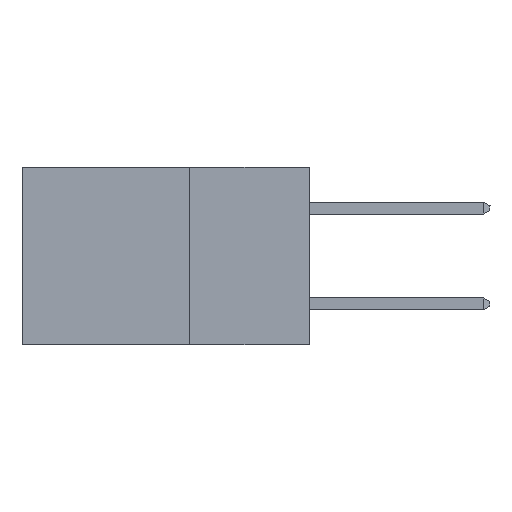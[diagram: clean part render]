
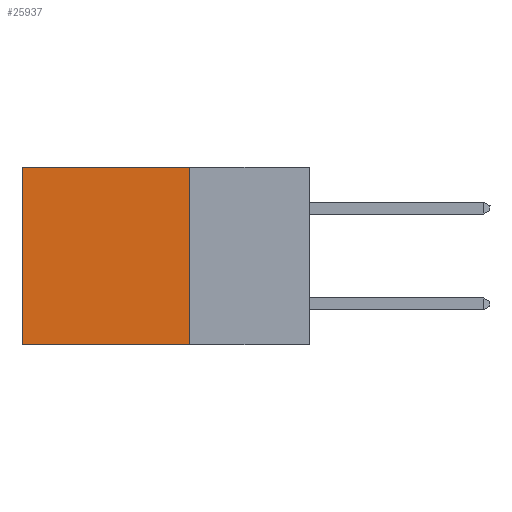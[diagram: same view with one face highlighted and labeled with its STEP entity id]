
A CAD part, left-side view. The second image highlights one B-rep face of the part: STEP entity #25937.
In plain terms, the highlighted planar face has unit normal (-1, 0, 0).
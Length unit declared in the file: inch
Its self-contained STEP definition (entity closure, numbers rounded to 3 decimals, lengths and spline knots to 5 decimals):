
#887 = CARTESIAN_POINT ( 'NONE',  ( 0.2875, 0.25, 0. ) ) ;
#1950 = ORIENTED_EDGE ( 'NONE', *, *, #26668, .T. ) ;
#3660 = VECTOR ( 'NONE', #9837, 39.37008 ) ;
#6089 = EDGE_LOOP ( 'NONE', ( #31651, #23445, #15023, #1950 ) ) ;
#6112 = LINE ( 'NONE', #8741, #6908 ) ;
#6908 = VECTOR ( 'NONE', #26949, 39.37008 ) ;
#7460 = CARTESIAN_POINT ( 'NONE',  ( 0.2875, 0.6, 0. ) ) ;
#8358 = VERTEX_POINT ( 'NONE', #23331 ) ;
#8589 = VERTEX_POINT ( 'NONE', #19470 ) ;
#8741 = CARTESIAN_POINT ( 'NONE',  ( 0.2875, 0.25, -0.37 ) ) ;
#9783 = FACE_OUTER_BOUND ( 'NONE', #6089, .T. ) ;
#9837 = DIRECTION ( 'NONE',  ( 0., 1., 0. ) ) ;
#12828 = CARTESIAN_POINT ( 'NONE',  ( 0.2875, 0.25, -0.37 ) ) ;
#12877 = LINE ( 'NONE', #25206, #3660 ) ;
#13522 = LINE ( 'NONE', #38189, #35384 ) ;
#14316 = LINE ( 'NONE', #7460, #39404 ) ;
#15023 = ORIENTED_EDGE ( 'NONE', *, *, #29424, .F. ) ;
#17444 = EDGE_CURVE ( 'NONE', #27073, #8589, #6112, .T. ) ;
#17999 = VERTEX_POINT ( 'NONE', #34729 ) ;
#19470 = CARTESIAN_POINT ( 'NONE',  ( 0.2875, 0.6, -0.37 ) ) ;
#19994 = DIRECTION ( 'NONE',  ( 0., 0., -1. ) ) ;
#23217 = DIRECTION ( 'NONE',  ( 0., 0., -1. ) ) ;
#23331 = CARTESIAN_POINT ( 'NONE',  ( 0.2875, 0.25, 0. ) ) ;
#23445 = ORIENTED_EDGE ( 'NONE', *, *, #17444, .F. ) ;
#25146 = DIRECTION ( 'NONE',  ( 1., 0., 0. ) ) ;
#25206 = CARTESIAN_POINT ( 'NONE',  ( 0.2875, 0.25, 0. ) ) ;
#25548 = PLANE ( 'NONE',  #26853 ) ;
#25937 = ADVANCED_FACE ( 'NONE', ( #9783 ), #25548, .F. ) ;
#26668 = EDGE_CURVE ( 'NONE', #8358, #17999, #12877, .T. ) ;
#26853 = AXIS2_PLACEMENT_3D ( 'NONE', #887, #25146, #37484 ) ;
#26949 = DIRECTION ( 'NONE',  ( 0., 1., 0. ) ) ;
#27073 = VERTEX_POINT ( 'NONE', #12828 ) ;
#29424 = EDGE_CURVE ( 'NONE', #8358, #27073, #13522, .T. ) ;
#31651 = ORIENTED_EDGE ( 'NONE', *, *, #32586, .T. ) ;
#32586 = EDGE_CURVE ( 'NONE', #17999, #8589, #14316, .T. ) ;
#34729 = CARTESIAN_POINT ( 'NONE',  ( 0.2875, 0.6, 0. ) ) ;
#35384 = VECTOR ( 'NONE', #19994, 39.37008 ) ;
#37484 = DIRECTION ( 'NONE',  ( 0., 0., -1. ) ) ;
#38189 = CARTESIAN_POINT ( 'NONE',  ( 0.2875, 0.25, 0. ) ) ;
#39404 = VECTOR ( 'NONE', #23217, 39.37008 ) ;
